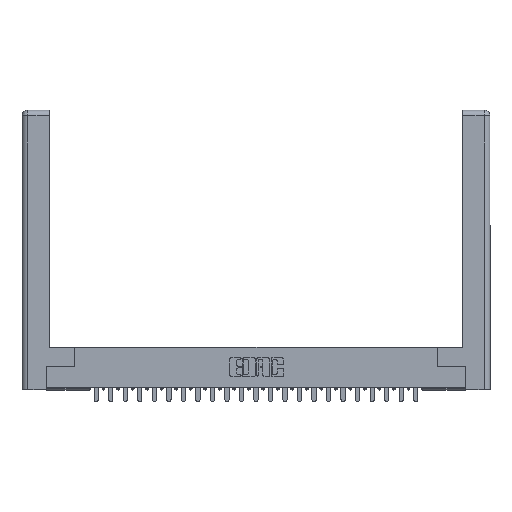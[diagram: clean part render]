
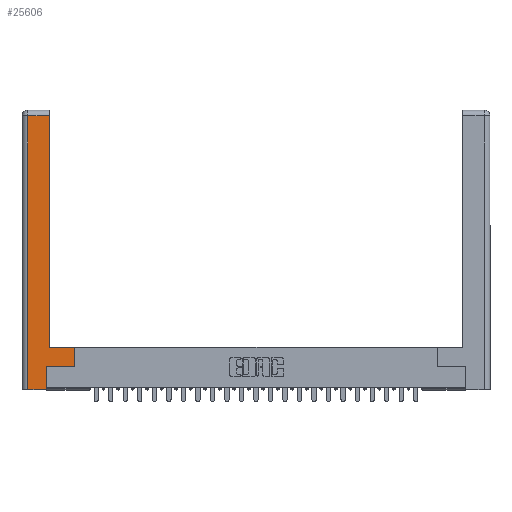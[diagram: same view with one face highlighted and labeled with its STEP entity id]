
A CAD part, top view. The second image highlights one B-rep face of the part: STEP entity #25606.
In plain terms, the highlighted planar face has unit normal (0, 0, 1).
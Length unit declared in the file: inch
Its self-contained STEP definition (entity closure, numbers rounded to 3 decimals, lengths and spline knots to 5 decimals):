
#323 = EDGE_CURVE ( 'NONE', #20359, #27613, #23946, .T. ) ;
#399 = AXIS2_PLACEMENT_3D ( 'NONE', #21692, #2990, #10301 ) ;
#868 = VECTOR ( 'NONE', #4446, 39.37008 ) ;
#1044 = ORIENTED_EDGE ( 'NONE', *, *, #18408, .T. ) ;
#1545 = CARTESIAN_POINT ( 'NONE',  ( 0.265, 0.245, 0. ) ) ;
#1945 = ORIENTED_EDGE ( 'NONE', *, *, #14981, .T. ) ;
#2128 = DIRECTION ( 'NONE',  ( 1., 0., 0. ) ) ;
#2465 = CARTESIAN_POINT ( 'NONE',  ( 0.565, 0.245, 0. ) ) ;
#2662 = LINE ( 'NONE', #17813, #5912 ) ;
#2901 = CARTESIAN_POINT ( 'NONE',  ( 0.265, 0.245, 0. ) ) ;
#2990 = DIRECTION ( 'NONE',  ( 0., 0., -1. ) ) ;
#3149 = VERTEX_POINT ( 'NONE', #2465 ) ;
#4157 = ORIENTED_EDGE ( 'NONE', *, *, #323, .T. ) ;
#4446 = DIRECTION ( 'NONE',  ( 0., 1., 0. ) ) ;
#4552 = CARTESIAN_POINT ( 'NONE',  ( 0.565, 0.45, 0. ) ) ;
#5912 = VECTOR ( 'NONE', #13477, 39.37008 ) ;
#6137 = CARTESIAN_POINT ( 'NONE',  ( 0.295, 0.45, 0. ) ) ;
#6524 = CARTESIAN_POINT ( 'NONE',  ( 0.265, 0., 0. ) ) ;
#6762 = CARTESIAN_POINT ( 'NONE',  ( 0.0615, 2.94, 0. ) ) ;
#7577 = EDGE_CURVE ( 'NONE', #24635, #19358, #8390, .T. ) ;
#8390 = LINE ( 'NONE', #28779, #11635 ) ;
#8765 = ORIENTED_EDGE ( 'NONE', *, *, #19853, .T. ) ;
#9116 = VECTOR ( 'NONE', #29516, 39.37008 ) ;
#10191 = PLANE ( 'NONE',  #399 ) ;
#10228 = EDGE_CURVE ( 'NONE', #16221, #28554, #2662, .T. ) ;
#10301 = DIRECTION ( 'NONE',  ( -1., 0., 0. ) ) ;
#10582 = ORIENTED_EDGE ( 'NONE', *, *, #23704, .T. ) ;
#11489 = CARTESIAN_POINT ( 'NONE',  ( 0.295, 3., 0. ) ) ;
#11635 = VECTOR ( 'NONE', #22034, 39.37008 ) ;
#12913 = CARTESIAN_POINT ( 'NONE',  ( 0.0615, 0., 0. ) ) ;
#13204 = DIRECTION ( 'NONE',  ( -1., 0., 0. ) ) ;
#13477 = DIRECTION ( 'NONE',  ( -1., 0., 0. ) ) ;
#13489 = VECTOR ( 'NONE', #2128, 39.37008 ) ;
#14107 = LINE ( 'NONE', #11489, #9116 ) ;
#14195 = LINE ( 'NONE', #25144, #13489 ) ;
#14981 = EDGE_CURVE ( 'NONE', #27613, #16221, #14107, .T. ) ;
#15251 = LINE ( 'NONE', #1545, #868 ) ;
#16221 = VERTEX_POINT ( 'NONE', #23881 ) ;
#16393 = CARTESIAN_POINT ( 'NONE',  ( 0.565, 0.45, 0. ) ) ;
#16503 = FACE_OUTER_BOUND ( 'NONE', #21405, .T. ) ;
#17094 = VECTOR ( 'NONE', #13204, 39.37008 ) ;
#17547 = VECTOR ( 'NONE', #24056, 39.37008 ) ;
#17813 = CARTESIAN_POINT ( 'NONE',  ( 0.0615, 2.94, 0. ) ) ;
#18408 = EDGE_CURVE ( 'NONE', #28554, #24635, #27619, .T. ) ;
#18448 = VECTOR ( 'NONE', #21208, 39.37008 ) ;
#19134 = CARTESIAN_POINT ( 'NONE',  ( 0.295, 0.45, 0. ) ) ;
#19252 = ORIENTED_EDGE ( 'NONE', *, *, #10228, .T. ) ;
#19358 = VERTEX_POINT ( 'NONE', #6524 ) ;
#19489 = LINE ( 'NONE', #16393, #18448 ) ;
#19853 = EDGE_CURVE ( 'NONE', #25417, #3149, #14195, .T. ) ;
#20359 = VERTEX_POINT ( 'NONE', #4552 ) ;
#21130 = EDGE_CURVE ( 'NONE', #19358, #25417, #15251, .T. ) ;
#21208 = DIRECTION ( 'NONE',  ( 0., 1., 0. ) ) ;
#21405 = EDGE_LOOP ( 'NONE', ( #1945, #19252, #1044, #26086, #29029, #8765, #10582, #4157 ) ) ;
#21692 = CARTESIAN_POINT ( 'NONE',  ( 0., 0., 0. ) ) ;
#22034 = DIRECTION ( 'NONE',  ( 1., 0., 0. ) ) ;
#23704 = EDGE_CURVE ( 'NONE', #3149, #20359, #19489, .T. ) ;
#23881 = CARTESIAN_POINT ( 'NONE',  ( 0.295, 2.94, 0. ) ) ;
#23946 = LINE ( 'NONE', #6137, #17094 ) ;
#24056 = DIRECTION ( 'NONE',  ( 0., -1., 0. ) ) ;
#24635 = VERTEX_POINT ( 'NONE', #29413 ) ;
#25144 = CARTESIAN_POINT ( 'NONE',  ( 0.565, 0.245, 0. ) ) ;
#25417 = VERTEX_POINT ( 'NONE', #2901 ) ;
#25606 = ADVANCED_FACE ( 'NONE', ( #16503 ), #10191, .F. ) ;
#26086 = ORIENTED_EDGE ( 'NONE', *, *, #7577, .T. ) ;
#27613 = VERTEX_POINT ( 'NONE', #19134 ) ;
#27619 = LINE ( 'NONE', #12913, #17547 ) ;
#28554 = VERTEX_POINT ( 'NONE', #6762 ) ;
#28779 = CARTESIAN_POINT ( 'NONE',  ( 0.265, 0., 0. ) ) ;
#29029 = ORIENTED_EDGE ( 'NONE', *, *, #21130, .T. ) ;
#29413 = CARTESIAN_POINT ( 'NONE',  ( 0.0615, 0., 0. ) ) ;
#29516 = DIRECTION ( 'NONE',  ( 0., 1., 0. ) ) ;
